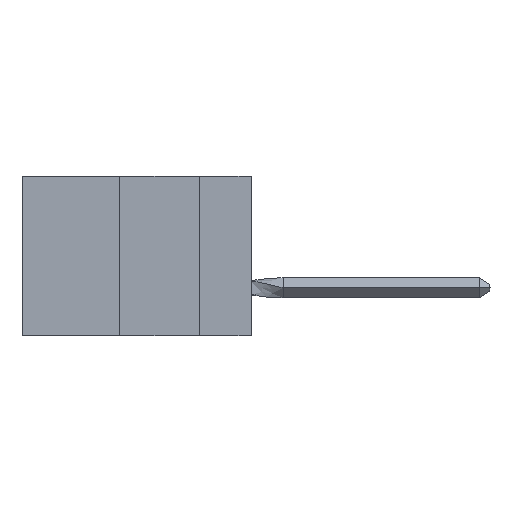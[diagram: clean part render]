
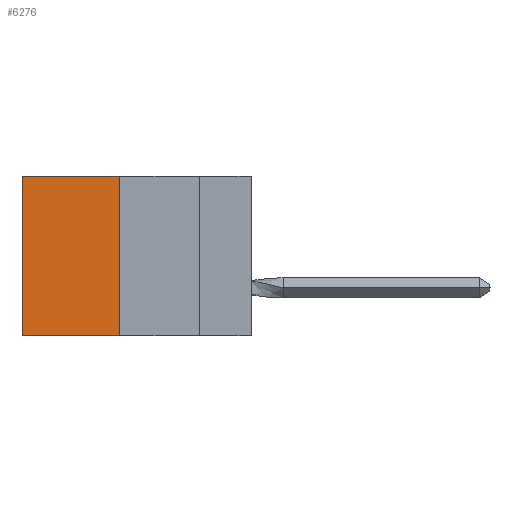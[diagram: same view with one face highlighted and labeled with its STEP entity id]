
A CAD part, left-side view. The second image highlights one B-rep face of the part: STEP entity #6276.
In plain terms, the highlighted planar face has unit normal (-1, 0, 0).
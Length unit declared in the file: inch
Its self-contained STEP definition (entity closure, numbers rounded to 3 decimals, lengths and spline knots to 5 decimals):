
#721 = VECTOR ( 'NONE', #1278, 39.37008 ) ;
#953 = ORIENTED_EDGE ( 'NONE', *, *, #17980, .T. ) ;
#1278 = DIRECTION ( 'NONE',  ( 0., 0., -1. ) ) ;
#1282 = DIRECTION ( 'NONE',  ( 0., 1., 0. ) ) ;
#2858 = DIRECTION ( 'NONE',  ( 1., 0., 0. ) ) ;
#3369 = DIRECTION ( 'NONE',  ( 0., 0., -1. ) ) ;
#4699 = EDGE_CURVE ( 'NONE', #18211, #16872, #15858, .T. ) ;
#5433 = EDGE_LOOP ( 'NONE', ( #953, #6066, #7202, #10441 ) ) ;
#6066 = ORIENTED_EDGE ( 'NONE', *, *, #4699, .F. ) ;
#6276 = ADVANCED_FACE ( 'NONE', ( #14113 ), #24070, .F. ) ;
#6410 = LINE ( 'NONE', #18643, #721 ) ;
#6522 = VECTOR ( 'NONE', #18437, 39.37008 ) ;
#7157 = DIRECTION ( 'NONE',  ( 0., 0., -1. ) ) ;
#7202 = ORIENTED_EDGE ( 'NONE', *, *, #8619, .F. ) ;
#8169 = CARTESIAN_POINT ( 'NONE',  ( 0.305, 0.413, 0. ) ) ;
#8619 = EDGE_CURVE ( 'NONE', #15449, #18211, #6410, .T. ) ;
#9363 = CARTESIAN_POINT ( 'NONE',  ( 0.305, 0.72, -0.5 ) ) ;
#10441 = ORIENTED_EDGE ( 'NONE', *, *, #11877, .T. ) ;
#11877 = EDGE_CURVE ( 'NONE', #15449, #14873, #23294, .T. ) ;
#12086 = CARTESIAN_POINT ( 'NONE',  ( 0.305, 0.72, -0.5 ) ) ;
#13522 = CARTESIAN_POINT ( 'NONE',  ( 0.305, 0.413, -0.5 ) ) ;
#14113 = FACE_OUTER_BOUND ( 'NONE', #5433, .T. ) ;
#14873 = VERTEX_POINT ( 'NONE', #20920 ) ;
#15231 = AXIS2_PLACEMENT_3D ( 'NONE', #13522, #2858, #7157 ) ;
#15449 = VERTEX_POINT ( 'NONE', #8169 ) ;
#15858 = LINE ( 'NONE', #22591, #6522 ) ;
#16872 = VERTEX_POINT ( 'NONE', #9363 ) ;
#17980 = EDGE_CURVE ( 'NONE', #14873, #16872, #26020, .T. ) ;
#18211 = VERTEX_POINT ( 'NONE', #21507 ) ;
#18437 = DIRECTION ( 'NONE',  ( 0., 1., 0. ) ) ;
#18643 = CARTESIAN_POINT ( 'NONE',  ( 0.305, 0.413, -0.5 ) ) ;
#18646 = CARTESIAN_POINT ( 'NONE',  ( 0.305, 0.413, 0. ) ) ;
#20920 = CARTESIAN_POINT ( 'NONE',  ( 0.305, 0.72, 0. ) ) ;
#21507 = CARTESIAN_POINT ( 'NONE',  ( 0.305, 0.413, -0.5 ) ) ;
#22591 = CARTESIAN_POINT ( 'NONE',  ( 0.305, 0.413, -0.5 ) ) ;
#23294 = LINE ( 'NONE', #18646, #24631 ) ;
#24070 = PLANE ( 'NONE',  #15231 ) ;
#24631 = VECTOR ( 'NONE', #1282, 39.37008 ) ;
#25701 = VECTOR ( 'NONE', #3369, 39.37008 ) ;
#26020 = LINE ( 'NONE', #12086, #25701 ) ;
